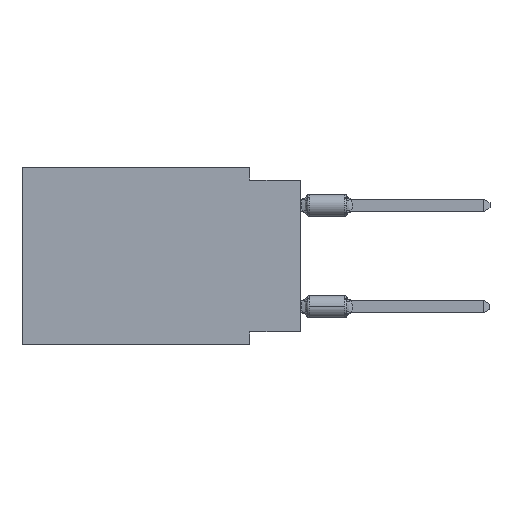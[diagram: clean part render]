
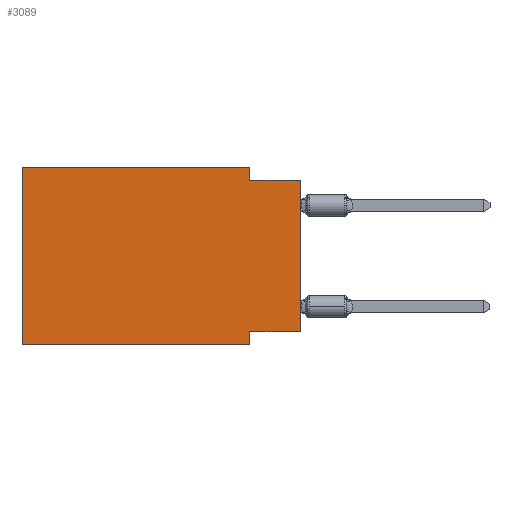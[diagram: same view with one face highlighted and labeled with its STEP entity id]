
A CAD part, left-side view. The second image highlights one B-rep face of the part: STEP entity #3089.
In plain terms, the highlighted planar face has unit normal (-1, 0, 0).
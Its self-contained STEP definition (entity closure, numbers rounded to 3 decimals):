
#260 = ORIENTED_EDGE ( 'NONE', *, *, #4063, .F. ) ;
#909 = PLANE ( 'NONE',  #10009 ) ;
#945 = VERTEX_POINT ( 'NONE', #10736 ) ;
#1075 = FACE_OUTER_BOUND ( 'NONE', #5701, .T. ) ;
#1533 = CARTESIAN_POINT ( 'NONE',  ( 0., 2.54, -8.89 ) ) ;
#2102 = ORIENTED_EDGE ( 'NONE', *, *, #10272, .F. ) ;
#2322 = DIRECTION ( 'NONE',  ( 0., -1., 0. ) ) ;
#2532 = CARTESIAN_POINT ( 'NONE',  ( 0., 0., -8.255 ) ) ;
#2604 = CARTESIAN_POINT ( 'NONE',  ( 0., 13.97, 0. ) ) ;
#2640 = DIRECTION ( 'NONE',  ( 0., 0., -1. ) ) ;
#2764 = VECTOR ( 'NONE', #12651, 1000. ) ;
#3089 = ADVANCED_FACE ( 'NONE', ( #1075 ), #909, .F. ) ;
#3212 = ORIENTED_EDGE ( 'NONE', *, *, #4023, .T. ) ;
#4023 = EDGE_CURVE ( 'NONE', #15762, #10664, #10842, .T. ) ;
#4063 = EDGE_CURVE ( 'NONE', #12726, #14887, #13363, .T. ) ;
#4488 = ORIENTED_EDGE ( 'NONE', *, *, #4796, .F. ) ;
#4796 = EDGE_CURVE ( 'NONE', #15762, #945, #6165, .T. ) ;
#4843 = CARTESIAN_POINT ( 'NONE',  ( 0., 0., -0.635 ) ) ;
#5516 = CARTESIAN_POINT ( 'NONE',  ( 0., 0., 0. ) ) ;
#5701 = EDGE_LOOP ( 'NONE', ( #3212, #15393, #2102, #260, #10493, #7418, #12420, #4488 ) ) ;
#5879 = LINE ( 'NONE', #15945, #8472 ) ;
#6104 = DIRECTION ( 'NONE',  ( 1., 0., 0. ) ) ;
#6165 = LINE ( 'NONE', #10051, #2764 ) ;
#6266 = VECTOR ( 'NONE', #14547, 1000. ) ;
#6354 = EDGE_CURVE ( 'NONE', #13877, #11091, #13990, .T. ) ;
#6357 = CARTESIAN_POINT ( 'NONE',  ( 0., 13.97, 0. ) ) ;
#6924 = VERTEX_POINT ( 'NONE', #10202 ) ;
#6933 = LINE ( 'NONE', #9370, #13064 ) ;
#7066 = VECTOR ( 'NONE', #7889, 1000. ) ;
#7071 = DIRECTION ( 'NONE',  ( 0., 0., 1. ) ) ;
#7279 = EDGE_CURVE ( 'NONE', #13877, #12726, #5879, .T. ) ;
#7418 = ORIENTED_EDGE ( 'NONE', *, *, #6354, .T. ) ;
#7889 = DIRECTION ( 'NONE',  ( 0., 0., 1. ) ) ;
#7936 = EDGE_CURVE ( 'NONE', #6924, #10664, #6933, .T. ) ;
#8305 = DIRECTION ( 'NONE',  ( 0., 0., -1. ) ) ;
#8472 = VECTOR ( 'NONE', #7071, 1000. ) ;
#8570 = CARTESIAN_POINT ( 'NONE',  ( 0., 2.54, 0. ) ) ;
#8625 = DIRECTION ( 'NONE',  ( 0., 0., -1. ) ) ;
#9276 = VECTOR ( 'NONE', #2322, 1000. ) ;
#9370 = CARTESIAN_POINT ( 'NONE',  ( 0., 0., -0.635 ) ) ;
#10009 = AXIS2_PLACEMENT_3D ( 'NONE', #6357, #6104, #8625 ) ;
#10051 = CARTESIAN_POINT ( 'NONE',  ( 0., 0., -8.255 ) ) ;
#10202 = CARTESIAN_POINT ( 'NONE',  ( 0., 2.54, -0.635 ) ) ;
#10272 = EDGE_CURVE ( 'NONE', #14887, #6924, #11840, .T. ) ;
#10493 = ORIENTED_EDGE ( 'NONE', *, *, #7279, .F. ) ;
#10586 = CARTESIAN_POINT ( 'NONE',  ( 0., 2.54, 0. ) ) ;
#10664 = VERTEX_POINT ( 'NONE', #4843 ) ;
#10736 = CARTESIAN_POINT ( 'NONE',  ( 0., 2.54, -8.255 ) ) ;
#10842 = LINE ( 'NONE', #5516, #7066 ) ;
#10855 = EDGE_CURVE ( 'NONE', #945, #11091, #15748, .T. ) ;
#11091 = VERTEX_POINT ( 'NONE', #12515 ) ;
#11261 = VECTOR ( 'NONE', #2640, 1000. ) ;
#11840 = LINE ( 'NONE', #10586, #11261 ) ;
#12420 = ORIENTED_EDGE ( 'NONE', *, *, #10855, .F. ) ;
#12515 = CARTESIAN_POINT ( 'NONE',  ( 0., 2.54, -8.89 ) ) ;
#12651 = DIRECTION ( 'NONE',  ( 0., 1., 0. ) ) ;
#12720 = CARTESIAN_POINT ( 'NONE',  ( 0., 13.97, -8.89 ) ) ;
#12726 = VERTEX_POINT ( 'NONE', #2604 ) ;
#13064 = VECTOR ( 'NONE', #14517, 1000. ) ;
#13174 = VECTOR ( 'NONE', #8305, 1000. ) ;
#13363 = LINE ( 'NONE', #15747, #6266 ) ;
#13877 = VERTEX_POINT ( 'NONE', #14862 ) ;
#13990 = LINE ( 'NONE', #12720, #9276 ) ;
#14517 = DIRECTION ( 'NONE',  ( 0., -1., 0. ) ) ;
#14547 = DIRECTION ( 'NONE',  ( 0., -1., 0. ) ) ;
#14862 = CARTESIAN_POINT ( 'NONE',  ( 0., 13.97, -8.89 ) ) ;
#14887 = VERTEX_POINT ( 'NONE', #8570 ) ;
#15393 = ORIENTED_EDGE ( 'NONE', *, *, #7936, .F. ) ;
#15747 = CARTESIAN_POINT ( 'NONE',  ( 0., 13.97, 0. ) ) ;
#15748 = LINE ( 'NONE', #1533, #13174 ) ;
#15762 = VERTEX_POINT ( 'NONE', #2532 ) ;
#15945 = CARTESIAN_POINT ( 'NONE',  ( 0., 13.97, 0. ) ) ;
